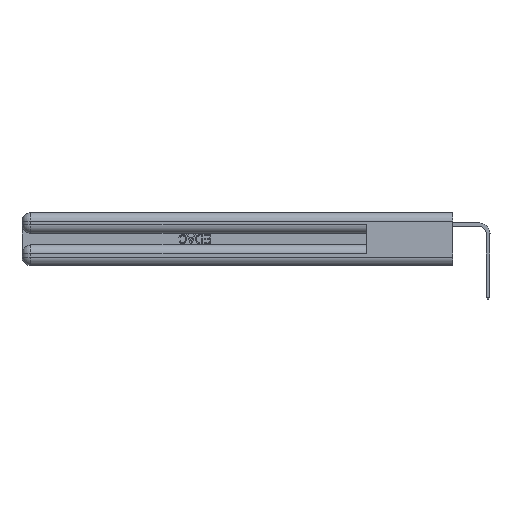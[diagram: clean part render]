
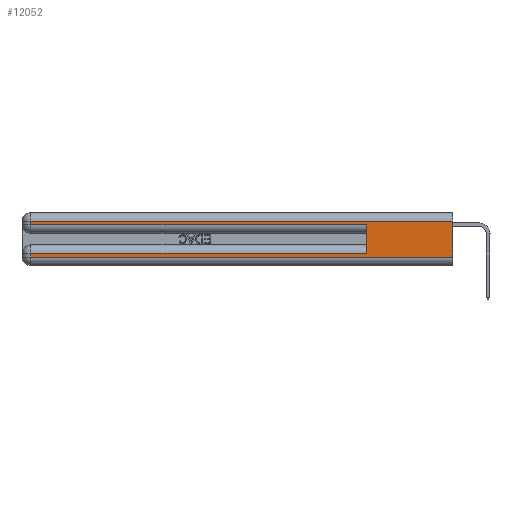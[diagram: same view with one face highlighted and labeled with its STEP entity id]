
A CAD part, left-side view. The second image highlights one B-rep face of the part: STEP entity #12052.
In plain terms, the highlighted planar face has unit normal (-1, 0, 0).
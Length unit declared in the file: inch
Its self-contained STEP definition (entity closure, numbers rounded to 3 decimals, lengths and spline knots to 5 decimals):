
#1435 = EDGE_CURVE ( 'NONE', #25320, #2985, #40310, .T. ) ;
#1737 = VERTEX_POINT ( 'NONE', #38197 ) ;
#2946 = ORIENTED_EDGE ( 'NONE', *, *, #35962, .F. ) ;
#2985 = VERTEX_POINT ( 'NONE', #40372 ) ;
#4732 = ORIENTED_EDGE ( 'NONE', *, *, #29693, .T. ) ;
#5440 = CARTESIAN_POINT ( 'NONE',  ( 0., 0., 0.31 ) ) ;
#6257 = DIRECTION ( 'NONE',  ( 0., 1., 0. ) ) ;
#6272 = EDGE_CURVE ( 'NONE', #7181, #19598, #26033, .T. ) ;
#6889 = VECTOR ( 'NONE', #13119, 39.37008 ) ;
#7153 = ORIENTED_EDGE ( 'NONE', *, *, #16323, .T. ) ;
#7181 = VERTEX_POINT ( 'NONE', #19805 ) ;
#7250 = VECTOR ( 'NONE', #18521, 39.37008 ) ;
#8970 = DIRECTION ( 'NONE',  ( 0., 0., -1. ) ) ;
#8972 = CARTESIAN_POINT ( 'NONE',  ( 0., 0., 0.37 ) ) ;
#9391 = CARTESIAN_POINT ( 'NONE',  ( 0., 0., 0.085 ) ) ;
#9594 = VECTOR ( 'NONE', #8970, 39.37008 ) ;
#9774 = ORIENTED_EDGE ( 'NONE', *, *, #36039, .T. ) ;
#12052 = ADVANCED_FACE ( 'NONE', ( #15530 ), #41112, .F. ) ;
#12212 = DIRECTION ( 'NONE',  ( 0., 0., -1. ) ) ;
#13119 = DIRECTION ( 'NONE',  ( 0., 0., -1. ) ) ;
#13733 = VERTEX_POINT ( 'NONE', #20793 ) ;
#15311 = CARTESIAN_POINT ( 'NONE',  ( 0., 2.94, 0.37 ) ) ;
#15530 = FACE_OUTER_BOUND ( 'NONE', #40123, .T. ) ;
#16044 = LINE ( 'NONE', #35662, #32226 ) ;
#16323 = EDGE_CURVE ( 'NONE', #19598, #1737, #16044, .T. ) ;
#16971 = DIRECTION ( 'NONE',  ( 0., 0., 1. ) ) ;
#18521 = DIRECTION ( 'NONE',  ( 0., 1., 0. ) ) ;
#19321 = EDGE_CURVE ( 'NONE', #13733, #36329, #25540, .T. ) ;
#19598 = VERTEX_POINT ( 'NONE', #23169 ) ;
#19753 = VECTOR ( 'NONE', #6257, 39.37008 ) ;
#19805 = CARTESIAN_POINT ( 'NONE',  ( 0., 2.94, 0.085 ) ) ;
#20793 = CARTESIAN_POINT ( 'NONE',  ( 0., 0., 0.31 ) ) ;
#21442 = VECTOR ( 'NONE', #22903, 39.37008 ) ;
#22457 = LINE ( 'NONE', #29367, #21442 ) ;
#22903 = DIRECTION ( 'NONE',  ( 0., -1., 0. ) ) ;
#23169 = CARTESIAN_POINT ( 'NONE',  ( 0., 2.94, 0.06 ) ) ;
#23560 = ORIENTED_EDGE ( 'NONE', *, *, #1435, .F. ) ;
#24170 = LINE ( 'NONE', #32507, #6889 ) ;
#25019 = VECTOR ( 'NONE', #28362, 39.37008 ) ;
#25320 = VERTEX_POINT ( 'NONE', #40321 ) ;
#25540 = LINE ( 'NONE', #5440, #7250 ) ;
#26033 = LINE ( 'NONE', #15311, #25019 ) ;
#27542 = ORIENTED_EDGE ( 'NONE', *, *, #19321, .T. ) ;
#28362 = DIRECTION ( 'NONE',  ( 0., 0., -1. ) ) ;
#28396 = CARTESIAN_POINT ( 'NONE',  ( 0., 0., 0.37 ) ) ;
#29315 = ORIENTED_EDGE ( 'NONE', *, *, #6272, .T. ) ;
#29336 = LINE ( 'NONE', #9391, #19753 ) ;
#29367 = CARTESIAN_POINT ( 'NONE',  ( 0., 0., 0.285 ) ) ;
#29621 = CARTESIAN_POINT ( 'NONE',  ( 0., 2.94, 0.285 ) ) ;
#29693 = EDGE_CURVE ( 'NONE', #39285, #2985, #22457, .T. ) ;
#29808 = CARTESIAN_POINT ( 'NONE',  ( 0., 0.6, 0.145 ) ) ;
#30792 = VECTOR ( 'NONE', #16971, 39.37008 ) ;
#31609 = DIRECTION ( 'NONE',  ( 1., 0., 0. ) ) ;
#32226 = VECTOR ( 'NONE', #38868, 39.37008 ) ;
#32362 = LINE ( 'NONE', #28396, #9594 ) ;
#32507 = CARTESIAN_POINT ( 'NONE',  ( 0., 2.94, 0.37 ) ) ;
#33209 = EDGE_CURVE ( 'NONE', #36329, #39285, #24170, .T. ) ;
#35662 = CARTESIAN_POINT ( 'NONE',  ( 0., 0., 0.06 ) ) ;
#35962 = EDGE_CURVE ( 'NONE', #13733, #1737, #32362, .T. ) ;
#36039 = EDGE_CURVE ( 'NONE', #25320, #7181, #29336, .T. ) ;
#36329 = VERTEX_POINT ( 'NONE', #39813 ) ;
#38197 = CARTESIAN_POINT ( 'NONE',  ( 0., 0., 0.06 ) ) ;
#38868 = DIRECTION ( 'NONE',  ( 0., -1., 0. ) ) ;
#38908 = ORIENTED_EDGE ( 'NONE', *, *, #33209, .T. ) ;
#39051 = AXIS2_PLACEMENT_3D ( 'NONE', #8972, #31609, #12212 ) ;
#39285 = VERTEX_POINT ( 'NONE', #29621 ) ;
#39813 = CARTESIAN_POINT ( 'NONE',  ( 0., 2.94, 0.31 ) ) ;
#40123 = EDGE_LOOP ( 'NONE', ( #2946, #27542, #38908, #4732, #23560, #9774, #29315, #7153 ) ) ;
#40310 = LINE ( 'NONE', #29808, #30792 ) ;
#40321 = CARTESIAN_POINT ( 'NONE',  ( 0., 0.6, 0.085 ) ) ;
#40372 = CARTESIAN_POINT ( 'NONE',  ( 0., 0.6, 0.285 ) ) ;
#41112 = PLANE ( 'NONE',  #39051 ) ;
